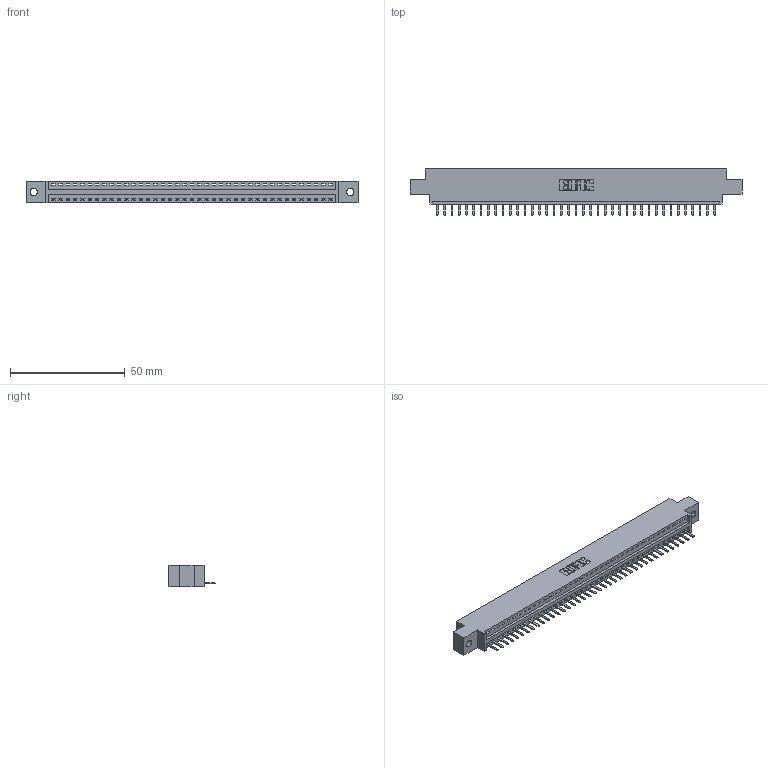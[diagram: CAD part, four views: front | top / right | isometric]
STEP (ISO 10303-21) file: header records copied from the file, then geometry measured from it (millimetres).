
FILE_DESCRIPTION (( 'STEP AP203' ), '1' );
FILE_NAME ('396-039-520-602.STEP', '2018-09-06T09:50:49', ( '' ), ( '' ), 'SwSTEP 2.0', 'SolidWorks 2016', '' );
FILE_SCHEMA (( 'CONFIG_CONTROL_DESIGN' ));
Length unit declared in the file: inch
Products named in the file (3): 396-039-520-602; 346 Part_0.170 Offset - 0.128 Dia; 345-292-001_345-293-120
Assembly tree (40 placements, depth 2):
  396-039-520-602
    346 Part_0.170 Offset - 0.128 Dia
    345-292-001_345-293-120  x39
Bounding box: 144.4 x 20.02 x 9.4 mm (x, y, z)
Volume: 13498 mm3; surface area: 16353 mm2
Topology: 40 solids, 40 shells, 2544 faces, 7517 edges, 4906 vertices
Faces by surface type: plane 1718, cylinder 826
Entity records: 24857 total; most frequent: CARTESIAN_POINT 4281, ORIENTED_EDGE 4242, DIRECTION 3767, EDGE_CURVE 2121, VECTOR 1829, LINE 1829, VERTEX_POINT 1410, AXIS2_PLACEMENT_3D 969
